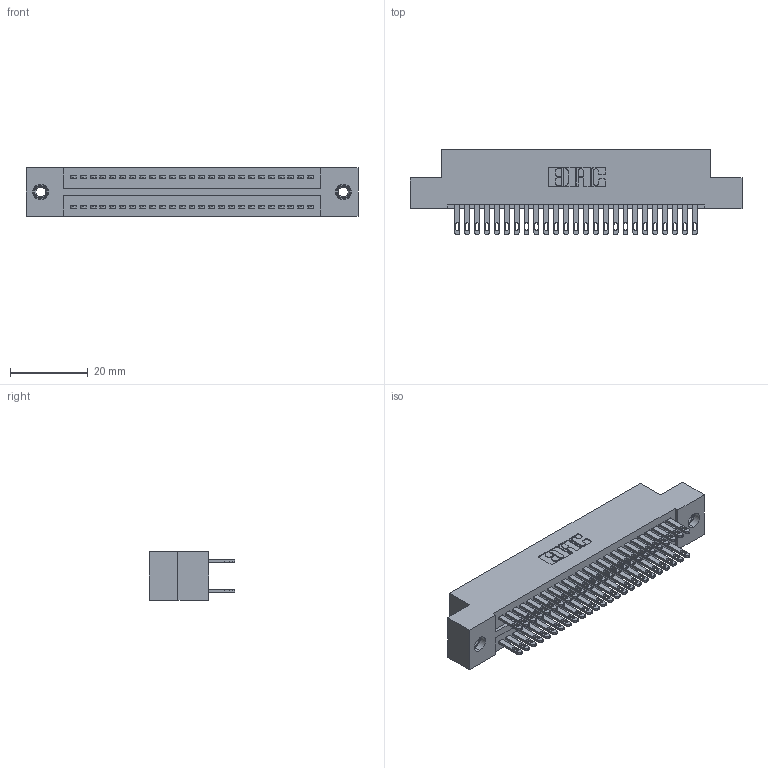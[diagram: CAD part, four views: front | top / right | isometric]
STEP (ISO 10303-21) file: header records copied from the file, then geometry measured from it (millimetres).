
FILE_DESCRIPTION (( 'STEP AP203' ), '1' );
FILE_NAME ('325-050-500-207.STEP', '2020-02-24T23:48:21', ( '' ), ( '' ), 'SwSTEP 2.0', 'SolidWorks 2016', '' );
FILE_SCHEMA (( 'CONFIG_CONTROL_DESIGN' ));
Length unit declared in the file: inch
Products named in the file (4): 325-050-500-207; 325 Part_TI; 345-250-001_345-250-005-103; 325-292-001_325-293-100
Assembly tree (53 placements, depth 2):
  325-050-500-207
    325 Part_TI
    325-292-001_325-293-100  x50
    345-250-001_345-250-005-103  x2
Bounding box: 85.22 x 21.84 x 12.45 mm (x, y, z)
Volume: 10987.9 mm3; surface area: 13445.3 mm2
Topology: 53 solids, 53 shells, 2574 faces, 7797 edges, 5190 vertices
Faces by surface type: plane 1602, cylinder 956, cone 12, torus 4
Entity records: 19398 total; most frequent: CARTESIAN_POINT 3217, ORIENTED_EDGE 3146, DIRECTION 2811, EDGE_CURVE 1573, VECTOR 1421, LINE 1421, VERTEX_POINT 1044, AXIS2_PLACEMENT_3D 695
